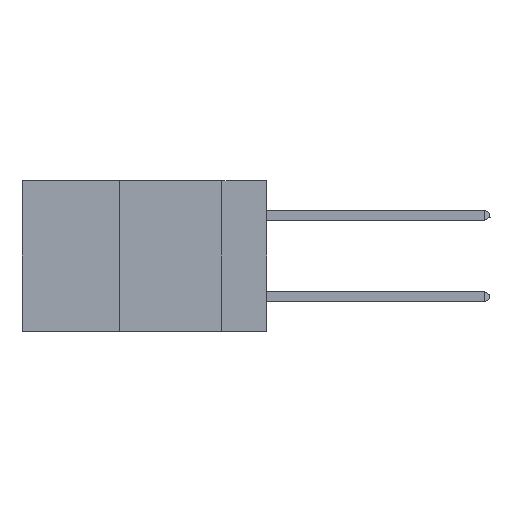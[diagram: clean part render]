
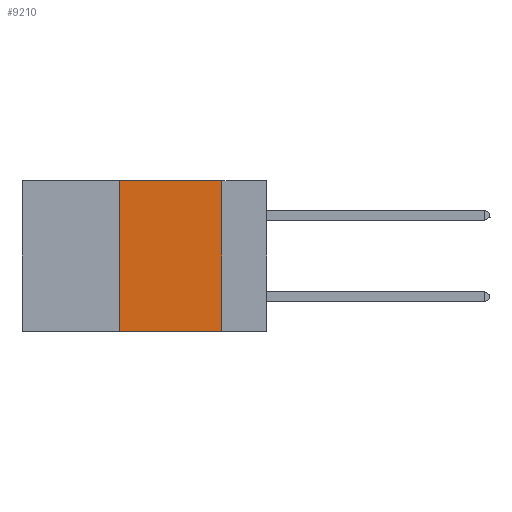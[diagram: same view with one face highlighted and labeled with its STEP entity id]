
A CAD part, left-side view. The second image highlights one B-rep face of the part: STEP entity #9210.
In plain terms, the highlighted planar face has unit normal (-1, 0, 0).
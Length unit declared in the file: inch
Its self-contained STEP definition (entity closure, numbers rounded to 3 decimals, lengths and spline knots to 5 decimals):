
#193 = LINE ( 'NONE', #10365, #9031 ) ;
#553 = CARTESIAN_POINT ( 'NONE',  ( 0., 0.36, 0. ) ) ;
#610 = LINE ( 'NONE', #553, #1763 ) ;
#967 = ORIENTED_EDGE ( 'NONE', *, *, #5079, .T. ) ;
#1763 = VECTOR ( 'NONE', #4656, 39.37008 ) ;
#1794 = AXIS2_PLACEMENT_3D ( 'NONE', #11339, #13297, #9158 ) ;
#2410 = EDGE_CURVE ( 'NONE', #4826, #5312, #610, .T. ) ;
#2612 = ORIENTED_EDGE ( 'NONE', *, *, #5799, .F. ) ;
#2872 = CARTESIAN_POINT ( 'NONE',  ( 0., 0.11, 0. ) ) ;
#3061 = ORIENTED_EDGE ( 'NONE', *, *, #13239, .F. ) ;
#4033 = CARTESIAN_POINT ( 'NONE',  ( 0., 0.11, 0. ) ) ;
#4394 = ORIENTED_EDGE ( 'NONE', *, *, #2410, .F. ) ;
#4656 = DIRECTION ( 'NONE',  ( 0., 0., 1. ) ) ;
#4826 = VERTEX_POINT ( 'NONE', #13262 ) ;
#4888 = LINE ( 'NONE', #2872, #6318 ) ;
#5015 = FACE_OUTER_BOUND ( 'NONE', #8778, .T. ) ;
#5079 = EDGE_CURVE ( 'NONE', #4826, #11612, #7626, .T. ) ;
#5312 = VERTEX_POINT ( 'NONE', #5419 ) ;
#5419 = CARTESIAN_POINT ( 'NONE',  ( 0., 0.36, 0. ) ) ;
#5775 = DIRECTION ( 'NONE',  ( 0., 0., -1. ) ) ;
#5799 = EDGE_CURVE ( 'NONE', #5312, #8736, #193, .T. ) ;
#6242 = CARTESIAN_POINT ( 'NONE',  ( 0., 0.11, -0.37 ) ) ;
#6318 = VECTOR ( 'NONE', #5775, 39.37008 ) ;
#6476 = DIRECTION ( 'NONE',  ( 0., -1., 0. ) ) ;
#6597 = CARTESIAN_POINT ( 'NONE',  ( 0., 0.6, -0.37 ) ) ;
#7626 = LINE ( 'NONE', #6597, #10758 ) ;
#7694 = DIRECTION ( 'NONE',  ( 0., -1., 0. ) ) ;
#8276 = PLANE ( 'NONE',  #1794 ) ;
#8736 = VERTEX_POINT ( 'NONE', #4033 ) ;
#8778 = EDGE_LOOP ( 'NONE', ( #3061, #2612, #4394, #967 ) ) ;
#9031 = VECTOR ( 'NONE', #6476, 39.37008 ) ;
#9158 = DIRECTION ( 'NONE',  ( 0., 0., -1. ) ) ;
#9210 = ADVANCED_FACE ( 'NONE', ( #5015 ), #8276, .F. ) ;
#10365 = CARTESIAN_POINT ( 'NONE',  ( 0., 0.6, 0. ) ) ;
#10758 = VECTOR ( 'NONE', #7694, 39.37008 ) ;
#11339 = CARTESIAN_POINT ( 'NONE',  ( 0., 0.6, 0. ) ) ;
#11612 = VERTEX_POINT ( 'NONE', #6242 ) ;
#13239 = EDGE_CURVE ( 'NONE', #8736, #11612, #4888, .T. ) ;
#13262 = CARTESIAN_POINT ( 'NONE',  ( 0., 0.36, -0.37 ) ) ;
#13297 = DIRECTION ( 'NONE',  ( 1., 0., 0. ) ) ;
